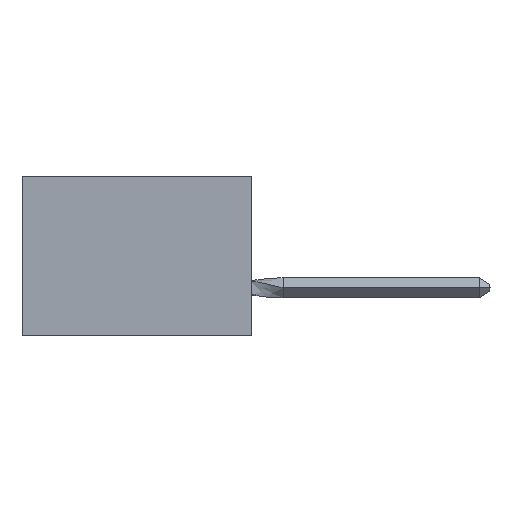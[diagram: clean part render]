
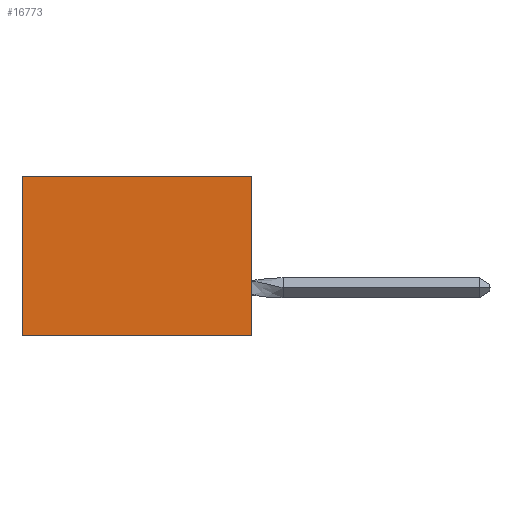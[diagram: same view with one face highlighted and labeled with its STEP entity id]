
A CAD part, left-side view. The second image highlights one B-rep face of the part: STEP entity #16773.
In plain terms, the highlighted planar face has unit normal (-1, 0, 0).
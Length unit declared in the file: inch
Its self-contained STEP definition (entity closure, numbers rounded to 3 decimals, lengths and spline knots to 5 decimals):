
#605 = EDGE_CURVE ( 'NONE', #3940, #13361, #21956, .T. ) ;
#1366 = ORIENTED_EDGE ( 'NONE', *, *, #5439, .T. ) ;
#2268 = VERTEX_POINT ( 'NONE', #15701 ) ;
#2944 = CARTESIAN_POINT ( 'NONE',  ( 0.305, 0., -0.5 ) ) ;
#3940 = VERTEX_POINT ( 'NONE', #31172 ) ;
#5439 = EDGE_CURVE ( 'NONE', #9010, #2268, #10205, .T. ) ;
#5480 = PLANE ( 'NONE',  #16447 ) ;
#5663 = CARTESIAN_POINT ( 'NONE',  ( 0.305, 0., -0.5 ) ) ;
#5819 = DIRECTION ( 'NONE',  ( 0., 1., 0. ) ) ;
#6562 = ORIENTED_EDGE ( 'NONE', *, *, #18594, .T. ) ;
#7400 = CARTESIAN_POINT ( 'NONE',  ( 0.305, 0.72, -0.5 ) ) ;
#8140 = LINE ( 'NONE', #30106, #20187 ) ;
#8518 = CARTESIAN_POINT ( 'NONE',  ( 0.305, 0., -0.5 ) ) ;
#8702 = VECTOR ( 'NONE', #17385, 39.37008 ) ;
#9010 = VERTEX_POINT ( 'NONE', #27881 ) ;
#9969 = LINE ( 'NONE', #26731, #28422 ) ;
#10205 = LINE ( 'NONE', #7400, #8702 ) ;
#10789 = DIRECTION ( 'NONE',  ( 0., 0., -1. ) ) ;
#11100 = ORIENTED_EDGE ( 'NONE', *, *, #18248, .F. ) ;
#11197 = ORIENTED_EDGE ( 'NONE', *, *, #605, .F. ) ;
#11201 = EDGE_LOOP ( 'NONE', ( #1366, #11100, #11197, #6562 ) ) ;
#13361 = VERTEX_POINT ( 'NONE', #8518 ) ;
#14719 = DIRECTION ( 'NONE',  ( 0., 1., 0. ) ) ;
#14767 = VECTOR ( 'NONE', #10789, 39.37008 ) ;
#15701 = CARTESIAN_POINT ( 'NONE',  ( 0.305, 0.72, -0.5 ) ) ;
#16447 = AXIS2_PLACEMENT_3D ( 'NONE', #2944, #17544, #19969 ) ;
#16773 = ADVANCED_FACE ( 'NONE', ( #25836 ), #5480, .F. ) ;
#17385 = DIRECTION ( 'NONE',  ( 0., 0., -1. ) ) ;
#17544 = DIRECTION ( 'NONE',  ( 1., 0., 0. ) ) ;
#18248 = EDGE_CURVE ( 'NONE', #13361, #2268, #8140, .T. ) ;
#18594 = EDGE_CURVE ( 'NONE', #3940, #9010, #9969, .T. ) ;
#19969 = DIRECTION ( 'NONE',  ( 0., 0., -1. ) ) ;
#20187 = VECTOR ( 'NONE', #5819, 39.37008 ) ;
#21956 = LINE ( 'NONE', #5663, #14767 ) ;
#25836 = FACE_OUTER_BOUND ( 'NONE', #11201, .T. ) ;
#26731 = CARTESIAN_POINT ( 'NONE',  ( 0.305, 0., 0. ) ) ;
#27881 = CARTESIAN_POINT ( 'NONE',  ( 0.305, 0.72, 0. ) ) ;
#28422 = VECTOR ( 'NONE', #14719, 39.37008 ) ;
#30106 = CARTESIAN_POINT ( 'NONE',  ( 0.305, 0., -0.5 ) ) ;
#31172 = CARTESIAN_POINT ( 'NONE',  ( 0.305, 0., 0. ) ) ;
